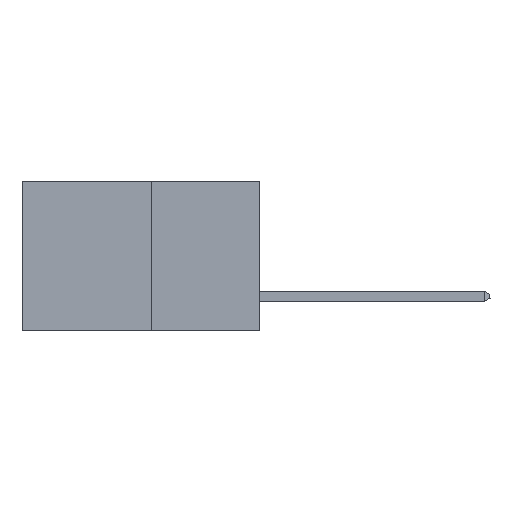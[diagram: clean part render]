
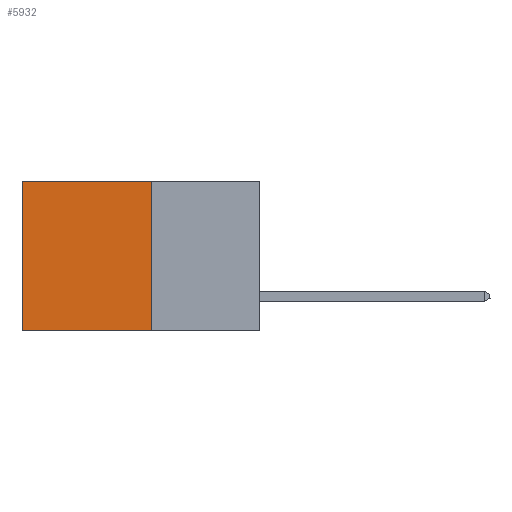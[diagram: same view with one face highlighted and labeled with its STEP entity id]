
A CAD part, left-side view. The second image highlights one B-rep face of the part: STEP entity #5932.
In plain terms, the highlighted planar face has unit normal (-1, 0, 0).
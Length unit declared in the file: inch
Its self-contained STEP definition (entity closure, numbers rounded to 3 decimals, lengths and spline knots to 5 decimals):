
#488 = CARTESIAN_POINT ( 'NONE',  ( 0.277, 0.27, -0.37 ) ) ;
#564 = ORIENTED_EDGE ( 'NONE', *, *, #22900, .F. ) ;
#2743 = EDGE_LOOP ( 'NONE', ( #28077, #29255, #564, #21485 ) ) ;
#2923 = CARTESIAN_POINT ( 'NONE',  ( 0.277, 0.27, 0. ) ) ;
#3291 = AXIS2_PLACEMENT_3D ( 'NONE', #8638, #8602, #8537 ) ;
#5826 = FACE_OUTER_BOUND ( 'NONE', #2743, .T. ) ;
#5932 = ADVANCED_FACE ( 'NONE', ( #5826 ), #8662, .F. ) ;
#8537 = DIRECTION ( 'NONE',  ( 0., 0., -1. ) ) ;
#8602 = DIRECTION ( 'NONE',  ( 1., 0., 0. ) ) ;
#8638 = CARTESIAN_POINT ( 'NONE',  ( 0.277, 0.27, -0.37 ) ) ;
#8662 = PLANE ( 'NONE',  #3291 ) ;
#12128 = CARTESIAN_POINT ( 'NONE',  ( 0.277, 0.27, -0.37 ) ) ;
#12676 = CARTESIAN_POINT ( 'NONE',  ( 0.277, 0.27, -0.37 ) ) ;
#12884 = EDGE_CURVE ( 'NONE', #29276, #19275, #21827, .T. ) ;
#12892 = EDGE_CURVE ( 'NONE', #14541, #19275, #27668, .T. ) ;
#14541 = VERTEX_POINT ( 'NONE', #29812 ) ;
#16568 = VECTOR ( 'NONE', #23071, 39.37008 ) ;
#17171 = VERTEX_POINT ( 'NONE', #25227 ) ;
#17353 = LINE ( 'NONE', #2923, #16568 ) ;
#17689 = LINE ( 'NONE', #12676, #30149 ) ;
#19275 = VERTEX_POINT ( 'NONE', #19801 ) ;
#19801 = CARTESIAN_POINT ( 'NONE',  ( 0.277, 0.59, -0.37 ) ) ;
#21024 = VECTOR ( 'NONE', #29547, 39.37008 ) ;
#21485 = ORIENTED_EDGE ( 'NONE', *, *, #22311, .T. ) ;
#21827 = LINE ( 'NONE', #12128, #28440 ) ;
#22311 = EDGE_CURVE ( 'NONE', #17171, #14541, #17353, .T. ) ;
#22900 = EDGE_CURVE ( 'NONE', #17171, #29276, #17689, .T. ) ;
#23071 = DIRECTION ( 'NONE',  ( 0., 1., 0. ) ) ;
#24555 = DIRECTION ( 'NONE',  ( 0., 1., 0. ) ) ;
#25101 = DIRECTION ( 'NONE',  ( 0., 0., -1. ) ) ;
#25227 = CARTESIAN_POINT ( 'NONE',  ( 0.277, 0.27, 0. ) ) ;
#26930 = CARTESIAN_POINT ( 'NONE',  ( 0.277, 0.59, -0.37 ) ) ;
#27668 = LINE ( 'NONE', #26930, #21024 ) ;
#28077 = ORIENTED_EDGE ( 'NONE', *, *, #12892, .T. ) ;
#28440 = VECTOR ( 'NONE', #24555, 39.37008 ) ;
#29255 = ORIENTED_EDGE ( 'NONE', *, *, #12884, .F. ) ;
#29276 = VERTEX_POINT ( 'NONE', #488 ) ;
#29547 = DIRECTION ( 'NONE',  ( 0., 0., -1. ) ) ;
#29812 = CARTESIAN_POINT ( 'NONE',  ( 0.277, 0.59, 0. ) ) ;
#30149 = VECTOR ( 'NONE', #25101, 39.37008 ) ;
